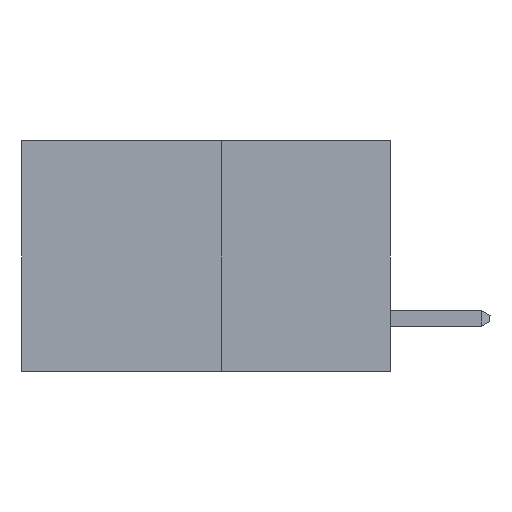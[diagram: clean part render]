
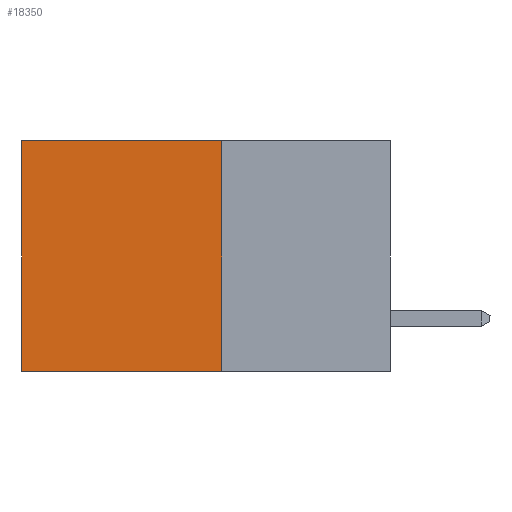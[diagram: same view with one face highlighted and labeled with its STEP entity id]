
A CAD part, left-side view. The second image highlights one B-rep face of the part: STEP entity #18350.
In plain terms, the highlighted planar face has unit normal (-1, 0, 0).
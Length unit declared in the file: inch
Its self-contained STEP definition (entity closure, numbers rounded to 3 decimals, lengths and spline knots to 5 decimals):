
#657 = DIRECTION ( 'NONE',  ( 0., 0., -1. ) ) ;
#749 = CARTESIAN_POINT ( 'NONE',  ( 0.277, 0.27, -0.37 ) ) ;
#842 = LINE ( 'NONE', #6871, #17596 ) ;
#1847 = LINE ( 'NONE', #11026, #14780 ) ;
#2652 = FACE_OUTER_BOUND ( 'NONE', #14153, .T. ) ;
#3172 = CARTESIAN_POINT ( 'NONE',  ( 0.277, 0.27, 0. ) ) ;
#3594 = VECTOR ( 'NONE', #657, 39.37008 ) ;
#3870 = VERTEX_POINT ( 'NONE', #14032 ) ;
#5229 = LINE ( 'NONE', #6874, #10127 ) ;
#5696 = ORIENTED_EDGE ( 'NONE', *, *, #7673, .T. ) ;
#5939 = DIRECTION ( 'NONE',  ( 0., 0., -1. ) ) ;
#6229 = ORIENTED_EDGE ( 'NONE', *, *, #8682, .F. ) ;
#6374 = EDGE_CURVE ( 'NONE', #9578, #3870, #842, .T. ) ;
#6871 = CARTESIAN_POINT ( 'NONE',  ( 0.277, 0.59, -0.37 ) ) ;
#6874 = CARTESIAN_POINT ( 'NONE',  ( 0.277, 0.27, -0.37 ) ) ;
#7673 = EDGE_CURVE ( 'NONE', #19967, #9578, #1847, .T. ) ;
#8682 = EDGE_CURVE ( 'NONE', #19967, #14211, #20664, .T. ) ;
#9000 = CARTESIAN_POINT ( 'NONE',  ( 0.277, 0.27, -0.37 ) ) ;
#9578 = VERTEX_POINT ( 'NONE', #19031 ) ;
#10127 = VECTOR ( 'NONE', #18103, 39.37008 ) ;
#10592 = ORIENTED_EDGE ( 'NONE', *, *, #15311, .F. ) ;
#10638 = DIRECTION ( 'NONE',  ( 0., 0., -1. ) ) ;
#11026 = CARTESIAN_POINT ( 'NONE',  ( 0.277, 0.27, 0. ) ) ;
#11092 = DIRECTION ( 'NONE',  ( 0., 1., 0. ) ) ;
#14032 = CARTESIAN_POINT ( 'NONE',  ( 0.277, 0.59, -0.37 ) ) ;
#14153 = EDGE_LOOP ( 'NONE', ( #18045, #10592, #6229, #5696 ) ) ;
#14211 = VERTEX_POINT ( 'NONE', #18339 ) ;
#14520 = AXIS2_PLACEMENT_3D ( 'NONE', #9000, #20111, #10638 ) ;
#14780 = VECTOR ( 'NONE', #11092, 39.37008 ) ;
#15311 = EDGE_CURVE ( 'NONE', #14211, #3870, #5229, .T. ) ;
#16947 = PLANE ( 'NONE',  #14520 ) ;
#17596 = VECTOR ( 'NONE', #5939, 39.37008 ) ;
#18045 = ORIENTED_EDGE ( 'NONE', *, *, #6374, .T. ) ;
#18103 = DIRECTION ( 'NONE',  ( 0., 1., 0. ) ) ;
#18339 = CARTESIAN_POINT ( 'NONE',  ( 0.277, 0.27, -0.37 ) ) ;
#18350 = ADVANCED_FACE ( 'NONE', ( #2652 ), #16947, .F. ) ;
#19031 = CARTESIAN_POINT ( 'NONE',  ( 0.277, 0.59, 0. ) ) ;
#19967 = VERTEX_POINT ( 'NONE', #3172 ) ;
#20111 = DIRECTION ( 'NONE',  ( 1., 0., 0. ) ) ;
#20664 = LINE ( 'NONE', #749, #3594 ) ;
